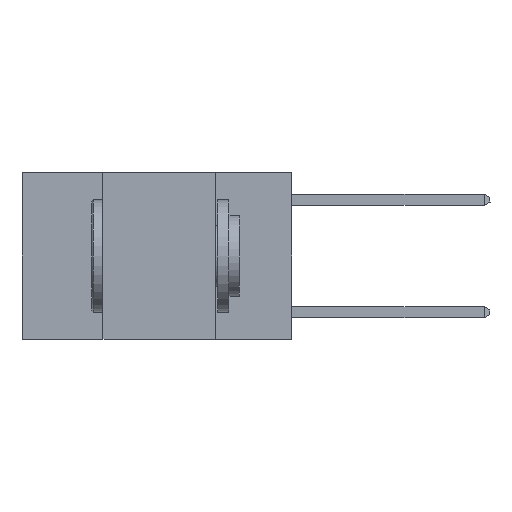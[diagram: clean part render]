
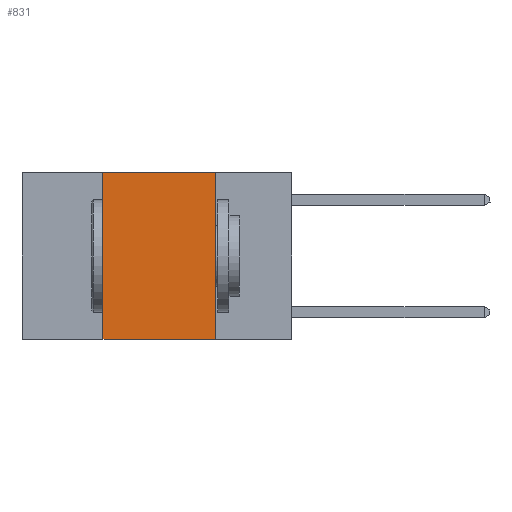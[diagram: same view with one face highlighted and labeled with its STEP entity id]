
A CAD part, left-side view. The second image highlights one B-rep face of the part: STEP entity #831.
In plain terms, the highlighted planar face has unit normal (-1, 0, 0).
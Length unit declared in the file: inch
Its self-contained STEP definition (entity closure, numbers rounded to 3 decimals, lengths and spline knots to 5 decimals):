
#74 = CARTESIAN_POINT ( 'NONE',  ( 0., 0.42, -0.37 ) ) ;
#408 = DIRECTION ( 'NONE',  ( 0., -1., 0. ) ) ;
#563 = CARTESIAN_POINT ( 'NONE',  ( 0., 0.42, 0. ) ) ;
#831 = ADVANCED_FACE ( 'NONE', ( #8108 ), #11123, .F. ) ;
#1840 = VECTOR ( 'NONE', #408, 39.37008 ) ;
#2299 = LINE ( 'NONE', #17911, #1840 ) ;
#2695 = DIRECTION ( 'NONE',  ( 1., 0., 0. ) ) ;
#2899 = VERTEX_POINT ( 'NONE', #11782 ) ;
#3403 = ORIENTED_EDGE ( 'NONE', *, *, #15021, .T. ) ;
#4167 = ORIENTED_EDGE ( 'NONE', *, *, #7288, .F. ) ;
#5082 = ORIENTED_EDGE ( 'NONE', *, *, #13073, .F. ) ;
#5670 = DIRECTION ( 'NONE',  ( 0., 0., -1. ) ) ;
#6232 = VECTOR ( 'NONE', #13555, 39.37008 ) ;
#7288 = EDGE_CURVE ( 'NONE', #16398, #14586, #8771, .T. ) ;
#7409 = DIRECTION ( 'NONE',  ( 0., -1., 0. ) ) ;
#7466 = CARTESIAN_POINT ( 'NONE',  ( 0., 0.17, 0. ) ) ;
#7660 = EDGE_CURVE ( 'NONE', #8862, #2899, #17760, .T. ) ;
#8108 = FACE_OUTER_BOUND ( 'NONE', #13469, .T. ) ;
#8771 = LINE ( 'NONE', #11426, #9227 ) ;
#8862 = VERTEX_POINT ( 'NONE', #7466 ) ;
#9227 = VECTOR ( 'NONE', #17157, 39.37008 ) ;
#11123 = PLANE ( 'NONE',  #11977 ) ;
#11426 = CARTESIAN_POINT ( 'NONE',  ( 0., 0.42, 0. ) ) ;
#11782 = CARTESIAN_POINT ( 'NONE',  ( 0., 0.17, -0.37 ) ) ;
#11977 = AXIS2_PLACEMENT_3D ( 'NONE', #13709, #2695, #5670 ) ;
#12099 = CARTESIAN_POINT ( 'NONE',  ( 0., 0.17, 0. ) ) ;
#13073 = EDGE_CURVE ( 'NONE', #14586, #8862, #2299, .T. ) ;
#13469 = EDGE_LOOP ( 'NONE', ( #18457, #5082, #4167, #3403 ) ) ;
#13555 = DIRECTION ( 'NONE',  ( 0., 0., -1. ) ) ;
#13709 = CARTESIAN_POINT ( 'NONE',  ( 0., 0.6, 0. ) ) ;
#14586 = VERTEX_POINT ( 'NONE', #563 ) ;
#15021 = EDGE_CURVE ( 'NONE', #16398, #2899, #17943, .T. ) ;
#16113 = CARTESIAN_POINT ( 'NONE',  ( 0., 0.6, -0.37 ) ) ;
#16398 = VERTEX_POINT ( 'NONE', #74 ) ;
#17157 = DIRECTION ( 'NONE',  ( 0., 0., 1. ) ) ;
#17760 = LINE ( 'NONE', #12099, #6232 ) ;
#17911 = CARTESIAN_POINT ( 'NONE',  ( 0., 0.6, 0. ) ) ;
#17943 = LINE ( 'NONE', #16113, #18386 ) ;
#18386 = VECTOR ( 'NONE', #7409, 39.37008 ) ;
#18457 = ORIENTED_EDGE ( 'NONE', *, *, #7660, .F. ) ;
